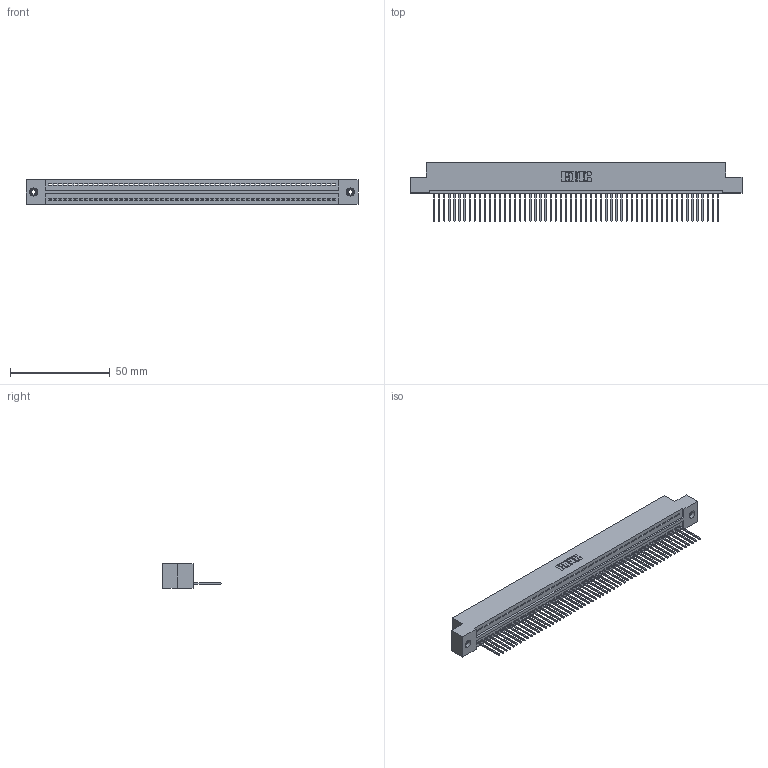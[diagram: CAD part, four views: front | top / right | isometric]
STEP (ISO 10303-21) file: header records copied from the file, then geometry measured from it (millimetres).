
FILE_DESCRIPTION (( 'STEP AP203' ), '1' );
FILE_NAME ('325-057-540-108.STEP', '2020-02-25T01:47:07', ( '' ), ( '' ), 'SwSTEP 2.0', 'SolidWorks 2016', '' );
FILE_SCHEMA (( 'CONFIG_CONTROL_DESIGN' ));
Length unit declared in the file: inch
Products named in the file (4): 325-057-540-108; 345-250-001_345-250-003-102; 325-292-001_325-293-140; 325 Part_TI
Assembly tree (60 placements, depth 2):
  325-057-540-108
    325 Part_TI
    325-292-001_325-293-140  x57
    345-250-001_345-250-003-102  x2
Bounding box: 166.5 x 29.46 x 12.45 mm (x, y, z)
Volume: 21325.7 mm3; surface area: 24139.2 mm2
Topology: 60 solids, 60 shells, 3480 faces, 10479 edges, 6902 vertices
Faces by surface type: plane 2496, cylinder 968, cone 12, torus 4
Entity records: 34110 total; most frequent: CARTESIAN_POINT 5864, ORIENTED_EDGE 5850, DIRECTION 4949, EDGE_CURVE 2925, VECTOR 2777, LINE 2777, VERTEX_POINT 1944, AXIS2_PLACEMENT_3D 1086
